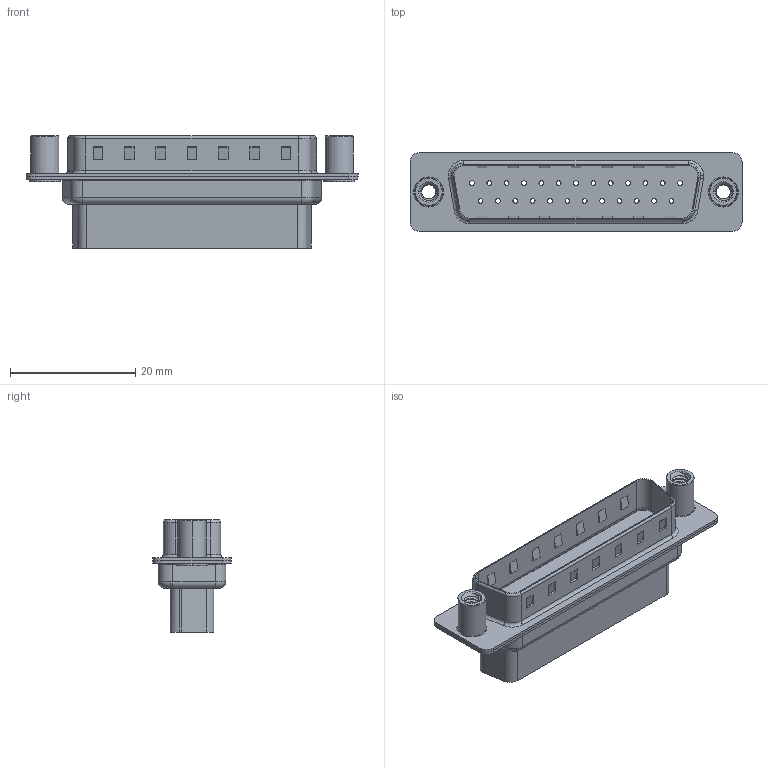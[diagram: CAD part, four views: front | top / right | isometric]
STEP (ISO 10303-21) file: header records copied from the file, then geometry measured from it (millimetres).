
FILE_DESCRIPTION (( 'STEP AP203' ), '1' );
FILE_NAME ('627-025-010-330.STEP', '2018-11-21T22:10:49', ( '' ), ( '' ), 'SwSTEP 2.0', 'SolidWorks 2016', '' );
FILE_SCHEMA (( 'CONFIG_CONTROL_DESIGN' ));
Length unit declared in the file: millimetre
Products named in the file (5): 627 Housing_25 HP; 627 Shell Front_25 Contacts; 627 Shell Rear_25 Contacts; 627 4-40 Threaded Standoff; 627-025-010-330
Assembly tree (5 placements, depth 2):
  627-025-010-330
    627 Housing_25 HP
    627 Shell Front_25 Contacts
    627 Shell Rear_25 Contacts
    627 4-40 Threaded Standoff  x2
Bounding box: 53 x 12.6 x 17.9 mm (x, y, z)
Volume: 3674 mm3; surface area: 6919.4 mm2
Topology: 5 solids, 5 shells, 610 faces, 1499 edges, 962 vertices
Faces by surface type: cylinder 315, plane 223, torus 50, cone 16, bspline 6
Entity records: 18938 total; most frequent: CARTESIAN_POINT 4638, DIRECTION 3026, ORIENTED_EDGE 2744, EDGE_CURVE 1372, AXIS2_PLACEMENT_3D 1160, VERTEX_POINT 880, EDGE_LOOP 712, VECTOR 706
